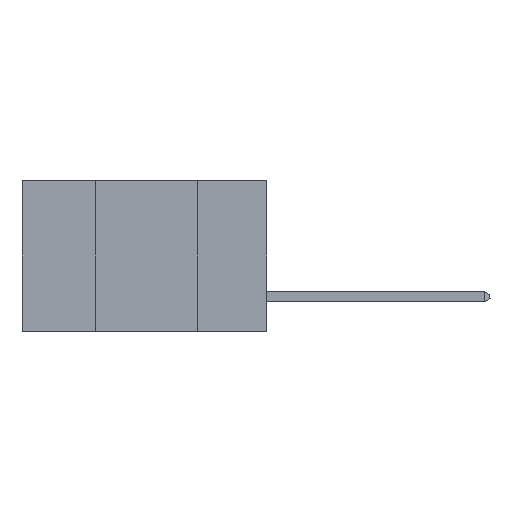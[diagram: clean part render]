
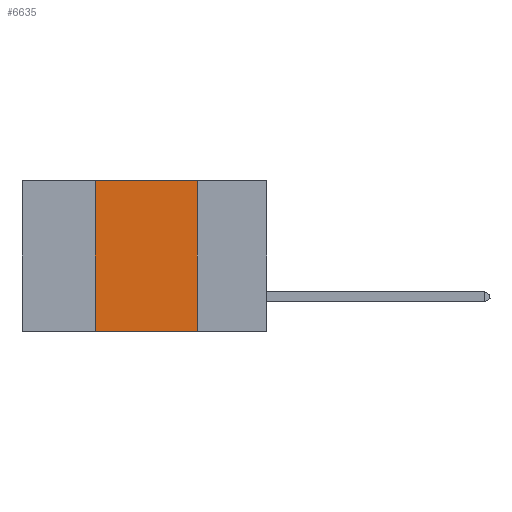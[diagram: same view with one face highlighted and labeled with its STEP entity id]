
A CAD part, left-side view. The second image highlights one B-rep face of the part: STEP entity #6635.
In plain terms, the highlighted planar face has unit normal (-1, 0, 0).
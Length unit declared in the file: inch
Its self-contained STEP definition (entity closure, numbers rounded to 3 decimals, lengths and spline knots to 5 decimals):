
#1118 = LINE ( 'NONE', #9737, #7609 ) ;
#1377 = CARTESIAN_POINT ( 'NONE',  ( 0., 0.6, -0.37 ) ) ;
#2058 = CARTESIAN_POINT ( 'NONE',  ( 0., 0.6, 0. ) ) ;
#2304 = ORIENTED_EDGE ( 'NONE', *, *, #11553, .F. ) ;
#3181 = EDGE_LOOP ( 'NONE', ( #2304, #9487, #6085, #14638 ) ) ;
#3543 = LINE ( 'NONE', #4877, #4630 ) ;
#3970 = CARTESIAN_POINT ( 'NONE',  ( 0., 0.17, -0.37 ) ) ;
#4630 = VECTOR ( 'NONE', #8595, 39.37008 ) ;
#4755 = CARTESIAN_POINT ( 'NONE',  ( 0., 0.42, -0.37 ) ) ;
#4877 = CARTESIAN_POINT ( 'NONE',  ( 0., 0.17, 0. ) ) ;
#4966 = DIRECTION ( 'NONE',  ( 0., -1., 0. ) ) ;
#5133 = DIRECTION ( 'NONE',  ( 0., -1., 0. ) ) ;
#5338 = EDGE_CURVE ( 'NONE', #5854, #7613, #14233, .T. ) ;
#5506 = VECTOR ( 'NONE', #4966, 39.37008 ) ;
#5854 = VERTEX_POINT ( 'NONE', #4755 ) ;
#6085 = ORIENTED_EDGE ( 'NONE', *, *, #6615, .F. ) ;
#6615 = EDGE_CURVE ( 'NONE', #5854, #7033, #11465, .T. ) ;
#6635 = ADVANCED_FACE ( 'NONE', ( #10740 ), #10300, .F. ) ;
#7033 = VERTEX_POINT ( 'NONE', #14164 ) ;
#7609 = VECTOR ( 'NONE', #5133, 39.37008 ) ;
#7613 = VERTEX_POINT ( 'NONE', #3970 ) ;
#7665 = EDGE_CURVE ( 'NONE', #7033, #11544, #1118, .T. ) ;
#8280 = CARTESIAN_POINT ( 'NONE',  ( 0., 0.17, 0. ) ) ;
#8595 = DIRECTION ( 'NONE',  ( 0., 0., -1. ) ) ;
#9061 = DIRECTION ( 'NONE',  ( 0., 0., 1. ) ) ;
#9487 = ORIENTED_EDGE ( 'NONE', *, *, #7665, .F. ) ;
#9737 = CARTESIAN_POINT ( 'NONE',  ( 0., 0.6, 0. ) ) ;
#10300 = PLANE ( 'NONE',  #13691 ) ;
#10740 = FACE_OUTER_BOUND ( 'NONE', #3181, .T. ) ;
#11465 = LINE ( 'NONE', #13750, #11846 ) ;
#11544 = VERTEX_POINT ( 'NONE', #8280 ) ;
#11553 = EDGE_CURVE ( 'NONE', #11544, #7613, #3543, .T. ) ;
#11846 = VECTOR ( 'NONE', #9061, 39.37008 ) ;
#13691 = AXIS2_PLACEMENT_3D ( 'NONE', #2058, #14806, #14960 ) ;
#13750 = CARTESIAN_POINT ( 'NONE',  ( 0., 0.42, 0. ) ) ;
#14164 = CARTESIAN_POINT ( 'NONE',  ( 0., 0.42, 0. ) ) ;
#14233 = LINE ( 'NONE', #1377, #5506 ) ;
#14638 = ORIENTED_EDGE ( 'NONE', *, *, #5338, .T. ) ;
#14806 = DIRECTION ( 'NONE',  ( 1., 0., 0. ) ) ;
#14960 = DIRECTION ( 'NONE',  ( 0., 0., -1. ) ) ;
